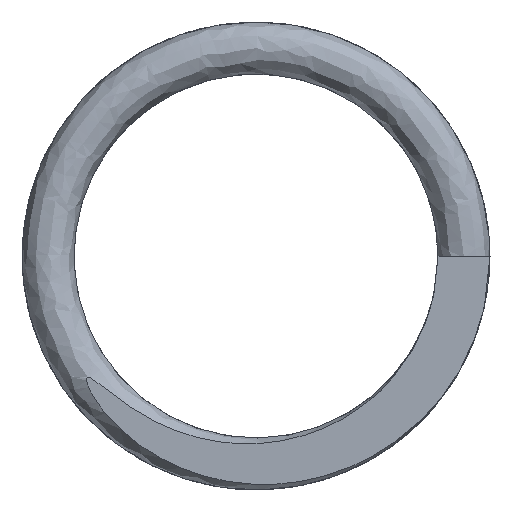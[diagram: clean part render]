
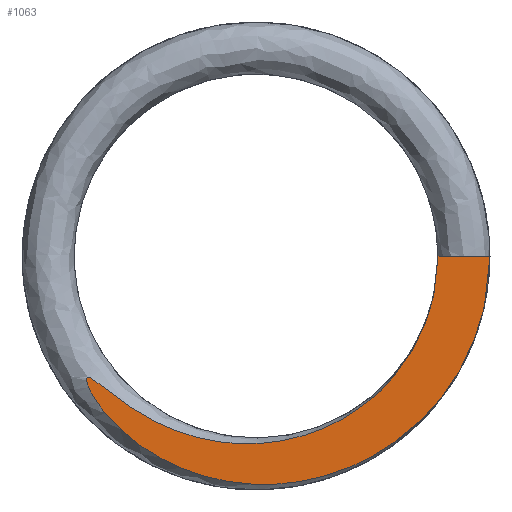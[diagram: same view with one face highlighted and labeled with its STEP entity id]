
A CAD part, front view. The second image highlights one B-rep face of the part: STEP entity #1063.
In plain terms, the highlighted planar face has unit normal (0, -1, 0).
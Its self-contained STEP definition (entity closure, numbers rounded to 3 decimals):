
#76 = CARTESIAN_POINT ( 'NONE',  ( 0., 0., -2.25 ) ) ;
#101 = CARTESIAN_POINT ( 'NONE',  ( 0.01, 0., -1.816 ) ) ;
#108 = CARTESIAN_POINT ( 'NONE',  ( -1.6, 0., -1.167 ) ) ;
#115 = CARTESIAN_POINT ( 'NONE',  ( -0.041, 0., -2.204 ) ) ;
#121 = CARTESIAN_POINT ( 'NONE',  ( 2.244, 0., -0.105 ) ) ;
#236 = DIRECTION ( 'NONE',  ( 1., 0., 0. ) ) ;
#254 = CARTESIAN_POINT ( 'NONE',  ( -0.625, 0., -1.74 ) ) ;
#263 = CARTESIAN_POINT ( 'NONE',  ( -1.626, 0., -1.172 ) ) ;
#269 = CARTESIAN_POINT ( 'NONE',  ( 0.583, 0., -2.146 ) ) ;
#315 = VERTEX_POINT ( 'NONE', #1164 ) ;
#385 = PLANE ( 'NONE',  #1291 ) ;
#400 = CARTESIAN_POINT ( 'NONE',  ( 1.75, 0., 0. ) ) ;
#409 = CARTESIAN_POINT ( 'NONE',  ( 1.738, 0., -0.213 ) ) ;
#419 = CARTESIAN_POINT ( 'NONE',  ( -1.111, 0., -1.519 ) ) ;
#427 = CARTESIAN_POINT ( 'NONE',  ( -1.629, 0., -1.192 ) ) ;
#434 = CARTESIAN_POINT ( 'NONE',  ( 1.164, 0., -1.912 ) ) ;
#558 = DIRECTION ( 'NONE',  ( 0., -1., 0. ) ) ;
#572 = CARTESIAN_POINT ( 'NONE',  ( 1.675, 0., -0.527 ) ) ;
#582 = CARTESIAN_POINT ( 'NONE',  ( -1.332, 0., -1.368 ) ) ;
#589 = CARTESIAN_POINT ( 'NONE',  ( -1.623, 0., -1.225 ) ) ;
#598 = CARTESIAN_POINT ( 'NONE',  ( 1.655, 0., -1.522 ) ) ;
#603 = B_SPLINE_CURVE_WITH_KNOTS ( 'NONE', 3,
 ( #400, #739, #409, #1582, #572, #1751, #750, #1916, #924, #2084, #1097, #101, #1257, #254, #1422, #419, #1593, #582, #1761, #760, #1926, #935, #2093, #1106, #108, #1265, #263, #1430, #427, #1600, #589, #1770, #768, #1932, #945, #2101, #1114, #115, #1273, #269, #1438, #434, #1608, #598, #1778, #776, #1940, #953, #2111, #1122, #121, #1281 ),
 .UNSPECIFIED., .F., .F.,
 ( 4, 2, 2, 2, 2, 2, 2, 2, 2, 2, 2, 2, 2, 2, 2, 2, 2, 2, 2, 2, 2, 2, 2, 2, 2, 4 ),
 ( 0., 0., 0.001, 0.001, 0.002, 0.003, 0.003, 0.004, 0.004, 0.004, 0.004, 0.005, 0.005, 0.005, 0.005, 0.005, 0.005, 0.005, 0.006, 0.007, 0.008, 0.008, 0.009, 0.01, 0.01, 0.01 ),
 .UNSPECIFIED. ) ;
#619 = CARTESIAN_POINT ( 'NONE',  ( 2., 0., 0. ) ) ;
#651 = ORIENTED_EDGE ( 'NONE', *, *, #2034, .T. ) ;
#700 = ORIENTED_EDGE ( 'NONE', *, *, #1641, .F. ) ;
#739 = CARTESIAN_POINT ( 'NONE',  ( 1.744, 0., -0.107 ) ) ;
#750 = CARTESIAN_POINT ( 'NONE',  ( 1.451, 0., -1.014 ) ) ;
#760 = CARTESIAN_POINT ( 'NONE',  ( -1.458, 0., -1.269 ) ) ;
#768 = CARTESIAN_POINT ( 'NONE',  ( -1.574, 0., -1.333 ) ) ;
#776 = CARTESIAN_POINT ( 'NONE',  ( 2.016, 0., -1.011 ) ) ;
#843 = EDGE_LOOP ( 'NONE', ( #651, #700 ) ) ;
#865 = VERTEX_POINT ( 'NONE', #1232 ) ;
#924 = CARTESIAN_POINT ( 'NONE',  ( 1.004, 0., -1.472 ) ) ;
#935 = CARTESIAN_POINT ( 'NONE',  ( -1.554, 0., -1.196 ) ) ;
#945 = CARTESIAN_POINT ( 'NONE',  ( -1.422, 0., -1.547 ) ) ;
#953 = CARTESIAN_POINT ( 'NONE',  ( 2.191, 0., -0.521 ) ) ;
#1063 = ADVANCED_FACE ( 'NONE', ( #1987 ), #385, .T. ) ;
#1097 = CARTESIAN_POINT ( 'NONE',  ( 0.428, 0., -1.748 ) ) ;
#1106 = CARTESIAN_POINT ( 'NONE',  ( -1.588, 0., -1.174 ) ) ;
#1114 = CARTESIAN_POINT ( 'NONE',  ( -0.657, 0., -2.108 ) ) ;
#1122 = CARTESIAN_POINT ( 'NONE',  ( 2.238, 0., -0.209 ) ) ;
#1164 = CARTESIAN_POINT ( 'NONE',  ( 1.75, 0., 0. ) ) ;
#1232 = CARTESIAN_POINT ( 'NONE',  ( 2.25, 0., 0. ) ) ;
#1257 = CARTESIAN_POINT ( 'NONE',  ( -0.208, 0., -1.814 ) ) ;
#1265 = CARTESIAN_POINT ( 'NONE',  ( -1.62, 0., -1.167 ) ) ;
#1273 = CARTESIAN_POINT ( 'NONE',  ( 0.172, 0., -2.205 ) ) ;
#1281 = CARTESIAN_POINT ( 'NONE',  ( 2.25, 0., 0. ) ) ;
#1291 = AXIS2_PLACEMENT_3D ( 'NONE', #76, #558, #1738 ) ;
#1422 = CARTESIAN_POINT ( 'NONE',  ( -0.83, 0., -1.668 ) ) ;
#1430 = CARTESIAN_POINT ( 'NONE',  ( -1.63, 0., -1.185 ) ) ;
#1438 = CARTESIAN_POINT ( 'NONE',  ( 0.786, 0., -2.086 ) ) ;
#1582 = CARTESIAN_POINT ( 'NONE',  ( 1.704, 0., -0.423 ) ) ;
#1593 = CARTESIAN_POINT ( 'NONE',  ( -1.201, 0., -1.462 ) ) ;
#1600 = CARTESIAN_POINT ( 'NONE',  ( -1.627, 0., -1.212 ) ) ;
#1608 = CARTESIAN_POINT ( 'NONE',  ( 1.341, 0., -1.797 ) ) ;
#1631 = LINE ( 'NONE', #619, #1878 ) ;
#1641 = EDGE_CURVE ( 'NONE', #315, #865, #1631, .T. ) ;
#1738 = DIRECTION ( 'NONE',  ( 0., 0., -1. ) ) ;
#1751 = CARTESIAN_POINT ( 'NONE',  ( 1.561, 0., -0.827 ) ) ;
#1761 = CARTESIAN_POINT ( 'NONE',  ( -1.374, 0., -1.335 ) ) ;
#1770 = CARTESIAN_POINT ( 'NONE',  ( -1.601, 0., -1.287 ) ) ;
#1778 = CARTESIAN_POINT ( 'NONE',  ( 1.791, 0., -1.365 ) ) ;
#1878 = VECTOR ( 'NONE', #236, 1000. ) ;
#1916 = CARTESIAN_POINT ( 'NONE',  ( 1.174, 0., -1.334 ) ) ;
#1926 = CARTESIAN_POINT ( 'NONE',  ( -1.5, 0., -1.235 ) ) ;
#1932 = CARTESIAN_POINT ( 'NONE',  ( -1.49, 0., -1.466 ) ) ;
#1940 = CARTESIAN_POINT ( 'NONE',  ( 2.103, 0., -0.822 ) ) ;
#1987 = FACE_OUTER_BOUND ( 'NONE', #843, .T. ) ;
#2034 = EDGE_CURVE ( 'NONE', #315, #865, #603, .T. ) ;
#2084 = CARTESIAN_POINT ( 'NONE',  ( 0.634, 0., -1.677 ) ) ;
#2093 = CARTESIAN_POINT ( 'NONE',  ( -1.565, 0., -1.188 ) ) ;
#2101 = CARTESIAN_POINT ( 'NONE',  ( -1.055, 0., -1.918 ) ) ;
#2111 = CARTESIAN_POINT ( 'NONE',  ( 2.212, 0., -0.417 ) ) ;
